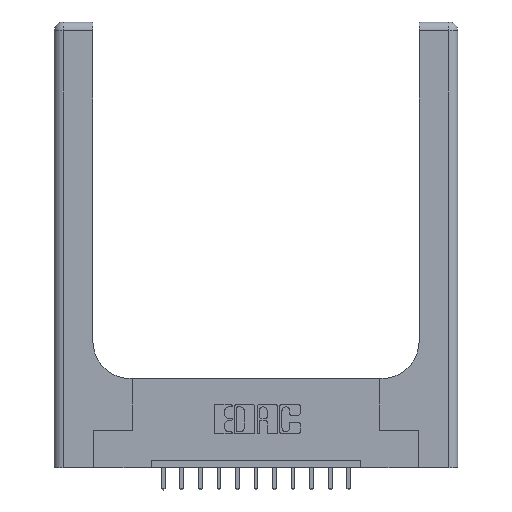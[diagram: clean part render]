
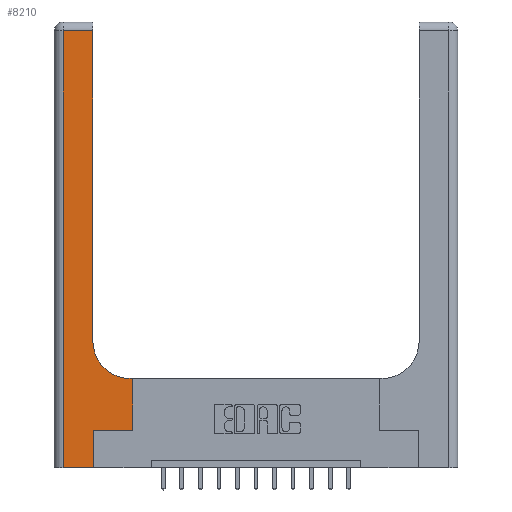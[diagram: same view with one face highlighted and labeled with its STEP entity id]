
A CAD part, top view. The second image highlights one B-rep face of the part: STEP entity #8210.
In plain terms, the highlighted planar face has unit normal (0, 0, 1).
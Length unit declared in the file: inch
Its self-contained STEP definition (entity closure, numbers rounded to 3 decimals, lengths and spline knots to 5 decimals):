
#85 = DIRECTION ( 'NONE',  ( 0., 1., 0. ) ) ;
#716 = EDGE_CURVE ( 'NONE', #2174, #4142, #13265, .T. ) ;
#2049 = ORIENTED_EDGE ( 'NONE', *, *, #3441, .T. ) ;
#2126 = ORIENTED_EDGE ( 'NONE', *, *, #6287, .T. ) ;
#2174 = VERTEX_POINT ( 'NONE', #14904 ) ;
#2319 = FACE_OUTER_BOUND ( 'NONE', #2514, .T. ) ;
#2365 = LINE ( 'NONE', #13717, #3144 ) ;
#2514 = EDGE_LOOP ( 'NONE', ( #4036, #4017, #4472, #7630, #15458, #2049, #6854, #3672, #2126 ) ) ;
#2584 = VERTEX_POINT ( 'NONE', #10692 ) ;
#2784 = EDGE_CURVE ( 'NONE', #4055, #9432, #12817, .T. ) ;
#3144 = VECTOR ( 'NONE', #13601, 39.37008 ) ;
#3239 = LINE ( 'NONE', #6965, #7760 ) ;
#3248 = CARTESIAN_POINT ( 'NONE',  ( 0.06, 3., 0.37 ) ) ;
#3415 = DIRECTION ( 'NONE',  ( 0., -1., 0. ) ) ;
#3441 = EDGE_CURVE ( 'NONE', #5176, #12976, #4408, .T. ) ;
#3672 = ORIENTED_EDGE ( 'NONE', *, *, #2784, .T. ) ;
#3752 = DIRECTION ( 'NONE',  ( 0., 0., -1. ) ) ;
#3893 = VERTEX_POINT ( 'NONE', #5284 ) ;
#4017 = ORIENTED_EDGE ( 'NONE', *, *, #716, .T. ) ;
#4036 = ORIENTED_EDGE ( 'NONE', *, *, #7317, .T. ) ;
#4055 = VERTEX_POINT ( 'NONE', #12833 ) ;
#4142 = VERTEX_POINT ( 'NONE', #14713 ) ;
#4236 = DIRECTION ( 'NONE',  ( 0., 0., -1. ) ) ;
#4408 = LINE ( 'NONE', #8726, #7152 ) ;
#4472 = ORIENTED_EDGE ( 'NONE', *, *, #8456, .T. ) ;
#4496 = DIRECTION ( 'NONE',  ( -1., 0., 0. ) ) ;
#5176 = VERTEX_POINT ( 'NONE', #10597 ) ;
#5284 = CARTESIAN_POINT ( 'NONE',  ( 0.265, 0., 0.37 ) ) ;
#5652 = CARTESIAN_POINT ( 'NONE',  ( 0., 3., 0.37 ) ) ;
#5802 = CARTESIAN_POINT ( 'NONE',  ( 0., 2.94, 0.37 ) ) ;
#6223 = AXIS2_PLACEMENT_3D ( 'NONE', #5652, #4236, #14352 ) ;
#6232 = VECTOR ( 'NONE', #85, 39.37008 ) ;
#6287 = EDGE_CURVE ( 'NONE', #9432, #14113, #14657, .T. ) ;
#6323 = CARTESIAN_POINT ( 'NONE',  ( 0.26, 3., 0.37 ) ) ;
#6854 = ORIENTED_EDGE ( 'NONE', *, *, #13639, .T. ) ;
#6965 = CARTESIAN_POINT ( 'NONE',  ( 0., 0., 0.37 ) ) ;
#7152 = VECTOR ( 'NONE', #14981, 39.37008 ) ;
#7289 = VECTOR ( 'NONE', #12980, 39.37008 ) ;
#7317 = EDGE_CURVE ( 'NONE', #14113, #2174, #9547, .T. ) ;
#7630 = ORIENTED_EDGE ( 'NONE', *, *, #10226, .T. ) ;
#7760 = VECTOR ( 'NONE', #15777, 39.37008 ) ;
#8012 = VECTOR ( 'NONE', #3415, 39.37008 ) ;
#8210 = ADVANCED_FACE ( 'NONE', ( #2319 ), #11832, .F. ) ;
#8255 = CARTESIAN_POINT ( 'NONE',  ( 0.528, 0.25, 0.37 ) ) ;
#8456 = EDGE_CURVE ( 'NONE', #4142, #2584, #11117, .T. ) ;
#8726 = CARTESIAN_POINT ( 'NONE',  ( 0.265, 0.25, 0.37 ) ) ;
#9432 = VERTEX_POINT ( 'NONE', #9674 ) ;
#9547 = LINE ( 'NONE', #6323, #6232 ) ;
#9674 = CARTESIAN_POINT ( 'NONE',  ( 0.51, 0.6, 0.37 ) ) ;
#9895 = DIRECTION ( 'NONE',  ( 1., 0., 0. ) ) ;
#10226 = EDGE_CURVE ( 'NONE', #2584, #3893, #3239, .T. ) ;
#10332 = CARTESIAN_POINT ( 'NONE',  ( 0.265, 0., 0.37 ) ) ;
#10363 = DIRECTION ( 'NONE',  ( -1., 0., 0. ) ) ;
#10597 = CARTESIAN_POINT ( 'NONE',  ( 0.265, 0.25, 0.37 ) ) ;
#10692 = CARTESIAN_POINT ( 'NONE',  ( 0.06, 0., 0.37 ) ) ;
#10852 = VECTOR ( 'NONE', #10363, 39.37008 ) ;
#11117 = LINE ( 'NONE', #3248, #8012 ) ;
#11832 = PLANE ( 'NONE',  #6223 ) ;
#11963 = LINE ( 'NONE', #10332, #7289 ) ;
#12324 = EDGE_CURVE ( 'NONE', #3893, #5176, #11963, .T. ) ;
#12509 = VECTOR ( 'NONE', #4496, 39.37008 ) ;
#12817 = LINE ( 'NONE', #12845, #10852 ) ;
#12833 = CARTESIAN_POINT ( 'NONE',  ( 0.528, 0.6, 0.37 ) ) ;
#12845 = CARTESIAN_POINT ( 'NONE',  ( 0.26, 0.6, 0.37 ) ) ;
#12976 = VERTEX_POINT ( 'NONE', #8255 ) ;
#12980 = DIRECTION ( 'NONE',  ( 0., 1., 0. ) ) ;
#13265 = LINE ( 'NONE', #5802, #12509 ) ;
#13583 = CARTESIAN_POINT ( 'NONE',  ( 0.26, 0.85, 0.37 ) ) ;
#13601 = DIRECTION ( 'NONE',  ( 0., 1., 0. ) ) ;
#13610 = CARTESIAN_POINT ( 'NONE',  ( 0.51, 0.85, 0.37 ) ) ;
#13639 = EDGE_CURVE ( 'NONE', #12976, #4055, #2365, .T. ) ;
#13717 = CARTESIAN_POINT ( 'NONE',  ( 0.528, 0.25, 0.37 ) ) ;
#14113 = VERTEX_POINT ( 'NONE', #13583 ) ;
#14352 = DIRECTION ( 'NONE',  ( -1., 0., 0. ) ) ;
#14657 = CIRCLE ( 'NONE', #15657, 0.25 ) ;
#14713 = CARTESIAN_POINT ( 'NONE',  ( 0.06, 2.94, 0.37 ) ) ;
#14904 = CARTESIAN_POINT ( 'NONE',  ( 0.26, 2.94, 0.37 ) ) ;
#14981 = DIRECTION ( 'NONE',  ( 1., 0., 0. ) ) ;
#15458 = ORIENTED_EDGE ( 'NONE', *, *, #12324, .T. ) ;
#15657 = AXIS2_PLACEMENT_3D ( 'NONE', #13610, #3752, #9895 ) ;
#15777 = DIRECTION ( 'NONE',  ( 1., 0., 0. ) ) ;
